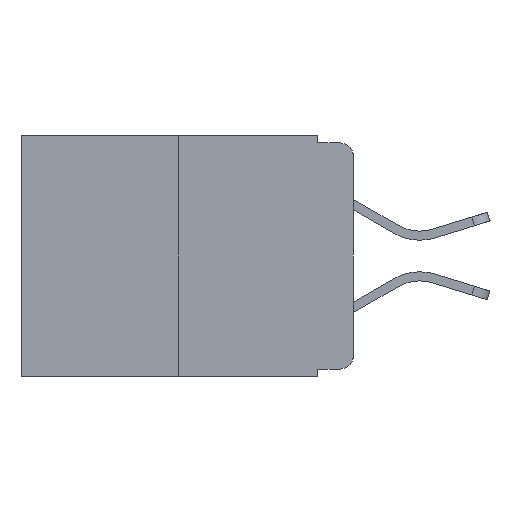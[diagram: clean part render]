
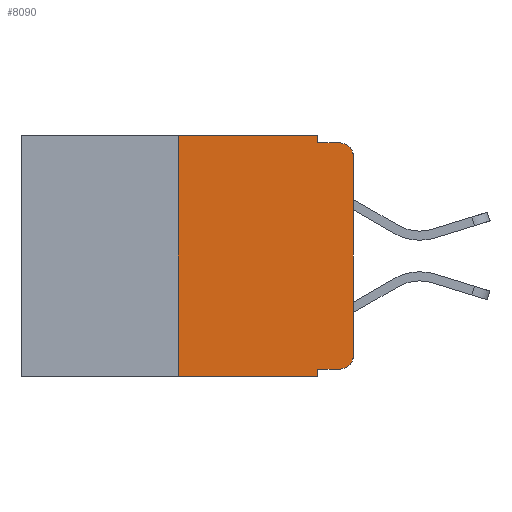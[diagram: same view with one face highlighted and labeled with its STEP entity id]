
A CAD part, left-side view. The second image highlights one B-rep face of the part: STEP entity #8090.
In plain terms, the highlighted planar face has unit normal (-1, 0, 0).
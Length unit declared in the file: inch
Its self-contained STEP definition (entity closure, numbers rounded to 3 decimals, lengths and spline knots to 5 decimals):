
#671 = ORIENTED_EDGE ( 'NONE', *, *, #17591, .T. ) ;
#949 = LINE ( 'NONE', #4018, #14442 ) ;
#1512 = CIRCLE ( 'NONE', #7098, 0.02 ) ;
#1836 = VERTEX_POINT ( 'NONE', #13692 ) ;
#1969 = EDGE_CURVE ( 'NONE', #14642, #8707, #15535, .T. ) ;
#2112 = VECTOR ( 'NONE', #13819, 39.37008 ) ;
#2197 = VECTOR ( 'NONE', #10050, 39.37008 ) ;
#3143 = DIRECTION ( 'NONE',  ( 0., 0., -1. ) ) ;
#3524 = DIRECTION ( 'NONE',  ( 0., -1., 0. ) ) ;
#3571 = VERTEX_POINT ( 'NONE', #14908 ) ;
#3595 = LINE ( 'NONE', #15262, #12616 ) ;
#3887 = ORIENTED_EDGE ( 'NONE', *, *, #15781, .F. ) ;
#3921 = ORIENTED_EDGE ( 'NONE', *, *, #1969, .F. ) ;
#4018 = CARTESIAN_POINT ( 'NONE',  ( 0., 0.473, 0. ) ) ;
#4197 = DIRECTION ( 'NONE',  ( 0., 0., 1. ) ) ;
#4369 = DIRECTION ( 'NONE',  ( 0., 0., -1. ) ) ;
#4771 = DIRECTION ( 'NONE',  ( -1., 0., 0. ) ) ;
#4843 = VERTEX_POINT ( 'NONE', #13285 ) ;
#5457 = EDGE_LOOP ( 'NONE', ( #671, #20628, #3887, #16726, #6569, #9257, #10588, #3921, #7969, #18047 ) ) ;
#5687 = CARTESIAN_POINT ( 'NONE',  ( 0., 0.051, -0.333 ) ) ;
#6100 = CARTESIAN_POINT ( 'NONE',  ( 0., 0.051, 0. ) ) ;
#6246 = CIRCLE ( 'NONE', #12159, 0.02 ) ;
#6467 = LINE ( 'NONE', #20494, #7268 ) ;
#6569 = ORIENTED_EDGE ( 'NONE', *, *, #7095, .F. ) ;
#6734 = VERTEX_POINT ( 'NONE', #9721 ) ;
#7095 = EDGE_CURVE ( 'NONE', #12900, #3571, #949, .T. ) ;
#7098 = AXIS2_PLACEMENT_3D ( 'NONE', #17570, #7652, #19233 ) ;
#7186 = LINE ( 'NONE', #5687, #19893 ) ;
#7198 = DIRECTION ( 'NONE',  ( 0., 0., 1. ) ) ;
#7268 = VECTOR ( 'NONE', #7198, 39.37008 ) ;
#7652 = DIRECTION ( 'NONE',  ( -1., 0., 0. ) ) ;
#7969 = ORIENTED_EDGE ( 'NONE', *, *, #13728, .T. ) ;
#8090 = ADVANCED_FACE ( 'NONE', ( #21120 ), #21502, .F. ) ;
#8321 = LINE ( 'NONE', #6100, #21026 ) ;
#8707 = VERTEX_POINT ( 'NONE', #21338 ) ;
#8735 = EDGE_CURVE ( 'NONE', #1836, #4843, #6246, .T. ) ;
#9257 = ORIENTED_EDGE ( 'NONE', *, *, #15504, .F. ) ;
#9297 = CARTESIAN_POINT ( 'NONE',  ( 0., 0.051, -0.01 ) ) ;
#9508 = VECTOR ( 'NONE', #4197, 39.37008 ) ;
#9721 = CARTESIAN_POINT ( 'NONE',  ( 0., 0.02, -0.333 ) ) ;
#10050 = DIRECTION ( 'NONE',  ( 0., -1., 0. ) ) ;
#10218 = CARTESIAN_POINT ( 'NONE',  ( 0., 0., -0.313 ) ) ;
#10274 = CARTESIAN_POINT ( 'NONE',  ( 0., 0.051, -0.333 ) ) ;
#10588 = ORIENTED_EDGE ( 'NONE', *, *, #16970, .T. ) ;
#10706 = EDGE_CURVE ( 'NONE', #3571, #19470, #8321, .T. ) ;
#10747 = LINE ( 'NONE', #11697, #2197 ) ;
#11610 = CARTESIAN_POINT ( 'NONE',  ( 0., 0.473, 0. ) ) ;
#11697 = CARTESIAN_POINT ( 'NONE',  ( 0., 0.473, -0.343 ) ) ;
#12159 = AXIS2_PLACEMENT_3D ( 'NONE', #14825, #4771, #16450 ) ;
#12616 = VECTOR ( 'NONE', #3524, 39.37008 ) ;
#12900 = VERTEX_POINT ( 'NONE', #13584 ) ;
#13276 = DIRECTION ( 'NONE',  ( 1., 0., 0. ) ) ;
#13285 = CARTESIAN_POINT ( 'NONE',  ( 0., 0.02, -0.01 ) ) ;
#13584 = CARTESIAN_POINT ( 'NONE',  ( 0., 0.25, 0. ) ) ;
#13692 = CARTESIAN_POINT ( 'NONE',  ( 0., 0., -0.03 ) ) ;
#13728 = EDGE_CURVE ( 'NONE', #14642, #6734, #7186, .T. ) ;
#13819 = DIRECTION ( 'NONE',  ( 0., 0., -1. ) ) ;
#14123 = VERTEX_POINT ( 'NONE', #10218 ) ;
#14442 = VECTOR ( 'NONE', #15736, 39.37008 ) ;
#14642 = VERTEX_POINT ( 'NONE', #10274 ) ;
#14825 = CARTESIAN_POINT ( 'NONE',  ( 0., 0.02, -0.03 ) ) ;
#14908 = CARTESIAN_POINT ( 'NONE',  ( 0., 0.051, 0. ) ) ;
#15262 = CARTESIAN_POINT ( 'NONE',  ( 0., 0.051, -0.01 ) ) ;
#15504 = EDGE_CURVE ( 'NONE', #17321, #12900, #18778, .T. ) ;
#15535 = LINE ( 'NONE', #17462, #2112 ) ;
#15736 = DIRECTION ( 'NONE',  ( 0., -1., 0. ) ) ;
#15781 = EDGE_CURVE ( 'NONE', #19470, #4843, #3595, .T. ) ;
#15915 = CARTESIAN_POINT ( 'NONE',  ( 0., 0.25, 0. ) ) ;
#16450 = DIRECTION ( 'NONE',  ( 0., 0., -1. ) ) ;
#16726 = ORIENTED_EDGE ( 'NONE', *, *, #10706, .F. ) ;
#16970 = EDGE_CURVE ( 'NONE', #17321, #8707, #10747, .T. ) ;
#17321 = VERTEX_POINT ( 'NONE', #19175 ) ;
#17335 = DIRECTION ( 'NONE',  ( 0., -1., 0. ) ) ;
#17462 = CARTESIAN_POINT ( 'NONE',  ( 0., 0.051, 0. ) ) ;
#17570 = CARTESIAN_POINT ( 'NONE',  ( 0., 0.02, -0.313 ) ) ;
#17591 = EDGE_CURVE ( 'NONE', #14123, #1836, #6467, .T. ) ;
#18047 = ORIENTED_EDGE ( 'NONE', *, *, #19475, .T. ) ;
#18778 = LINE ( 'NONE', #15915, #9508 ) ;
#19175 = CARTESIAN_POINT ( 'NONE',  ( 0., 0.25, -0.343 ) ) ;
#19233 = DIRECTION ( 'NONE',  ( 0., 0., -1. ) ) ;
#19470 = VERTEX_POINT ( 'NONE', #9297 ) ;
#19475 = EDGE_CURVE ( 'NONE', #6734, #14123, #1512, .T. ) ;
#19584 = AXIS2_PLACEMENT_3D ( 'NONE', #11610, #13276, #3143 ) ;
#19893 = VECTOR ( 'NONE', #17335, 39.37008 ) ;
#20494 = CARTESIAN_POINT ( 'NONE',  ( 0., 0., 0. ) ) ;
#20628 = ORIENTED_EDGE ( 'NONE', *, *, #8735, .T. ) ;
#21026 = VECTOR ( 'NONE', #4369, 39.37008 ) ;
#21120 = FACE_OUTER_BOUND ( 'NONE', #5457, .T. ) ;
#21338 = CARTESIAN_POINT ( 'NONE',  ( 0., 0.051, -0.343 ) ) ;
#21502 = PLANE ( 'NONE',  #19584 ) ;
